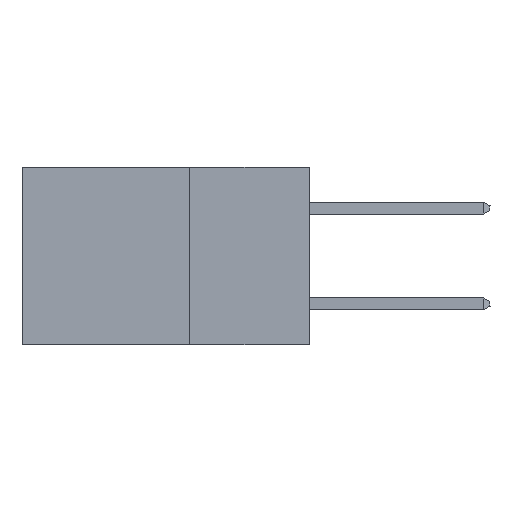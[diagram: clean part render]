
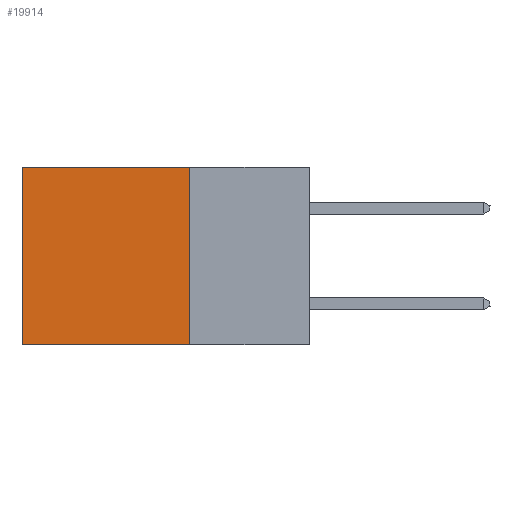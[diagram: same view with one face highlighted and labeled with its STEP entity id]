
A CAD part, left-side view. The second image highlights one B-rep face of the part: STEP entity #19914.
In plain terms, the highlighted planar face has unit normal (-1, 0, 0).
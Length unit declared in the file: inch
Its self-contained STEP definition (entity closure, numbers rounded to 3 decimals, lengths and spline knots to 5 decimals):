
#332 = VERTEX_POINT ( 'NONE', #13061 ) ;
#779 = EDGE_CURVE ( 'NONE', #332, #48206, #40325, .T. ) ;
#1735 = ORIENTED_EDGE ( 'NONE', *, *, #4620, .F. ) ;
#4464 = CARTESIAN_POINT ( 'NONE',  ( 0.2875, 0.6, 0. ) ) ;
#4620 = EDGE_CURVE ( 'NONE', #332, #40798, #35032, .T. ) ;
#5521 = CARTESIAN_POINT ( 'NONE',  ( 0.2875, 0.25, -0.37 ) ) ;
#7338 = EDGE_LOOP ( 'NONE', ( #19756, #12315, #1735, #33179 ) ) ;
#12274 = AXIS2_PLACEMENT_3D ( 'NONE', #39999, #48415, #32545 ) ;
#12315 = ORIENTED_EDGE ( 'NONE', *, *, #27342, .F. ) ;
#12814 = DIRECTION ( 'NONE',  ( 0., 0., -1. ) ) ;
#13061 = CARTESIAN_POINT ( 'NONE',  ( 0.2875, 0.25, 0. ) ) ;
#17090 = VECTOR ( 'NONE', #12814, 39.37008 ) ;
#18860 = DIRECTION ( 'NONE',  ( 0., 1., 0. ) ) ;
#19279 = PLANE ( 'NONE',  #12274 ) ;
#19756 = ORIENTED_EDGE ( 'NONE', *, *, #35221, .T. ) ;
#19914 = ADVANCED_FACE ( 'NONE', ( #44123 ), #19279, .F. ) ;
#27342 = EDGE_CURVE ( 'NONE', #40798, #49739, #39158, .T. ) ;
#28187 = CARTESIAN_POINT ( 'NONE',  ( 0.2875, 0.6, 0. ) ) ;
#28288 = DIRECTION ( 'NONE',  ( 0., 0., -1. ) ) ;
#28573 = VECTOR ( 'NONE', #18860, 39.37008 ) ;
#32545 = DIRECTION ( 'NONE',  ( 0., 0., -1. ) ) ;
#32600 = CARTESIAN_POINT ( 'NONE',  ( 0.2875, 0.25, 0. ) ) ;
#33179 = ORIENTED_EDGE ( 'NONE', *, *, #779, .T. ) ;
#35032 = LINE ( 'NONE', #32600, #44272 ) ;
#35221 = EDGE_CURVE ( 'NONE', #48206, #49739, #44275, .T. ) ;
#35865 = CARTESIAN_POINT ( 'NONE',  ( 0.2875, 0.25, -0.37 ) ) ;
#37150 = DIRECTION ( 'NONE',  ( 0., 1., 0. ) ) ;
#38041 = CARTESIAN_POINT ( 'NONE',  ( 0.2875, 0.25, 0. ) ) ;
#39158 = LINE ( 'NONE', #5521, #44678 ) ;
#39999 = CARTESIAN_POINT ( 'NONE',  ( 0.2875, 0.25, 0. ) ) ;
#40325 = LINE ( 'NONE', #38041, #28573 ) ;
#40798 = VERTEX_POINT ( 'NONE', #35865 ) ;
#44123 = FACE_OUTER_BOUND ( 'NONE', #7338, .T. ) ;
#44272 = VECTOR ( 'NONE', #28288, 39.37008 ) ;
#44275 = LINE ( 'NONE', #28187, #17090 ) ;
#44678 = VECTOR ( 'NONE', #37150, 39.37008 ) ;
#48206 = VERTEX_POINT ( 'NONE', #4464 ) ;
#48415 = DIRECTION ( 'NONE',  ( 1., 0., 0. ) ) ;
#49116 = CARTESIAN_POINT ( 'NONE',  ( 0.2875, 0.6, -0.37 ) ) ;
#49739 = VERTEX_POINT ( 'NONE', #49116 ) ;
